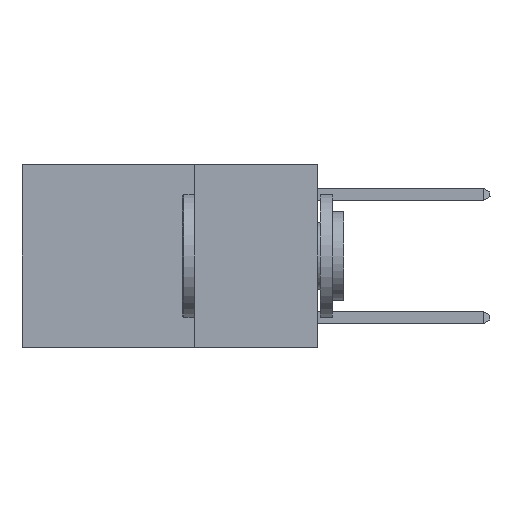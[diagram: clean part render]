
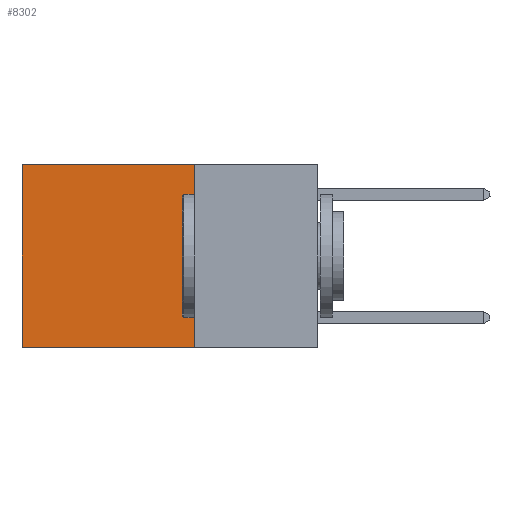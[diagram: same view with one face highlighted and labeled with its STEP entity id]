
A CAD part, left-side view. The second image highlights one B-rep face of the part: STEP entity #8302.
In plain terms, the highlighted planar face has unit normal (-1, 0, 0).
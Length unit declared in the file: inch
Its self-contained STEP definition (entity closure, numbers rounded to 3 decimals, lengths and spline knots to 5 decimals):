
#72 = LINE ( 'NONE', #10292, #3906 ) ;
#152 = VERTEX_POINT ( 'NONE', #9428 ) ;
#153 = ORIENTED_EDGE ( 'NONE', *, *, #1175, .T. ) ;
#186 = CARTESIAN_POINT ( 'NONE',  ( 0.2625, 0.6, 0. ) ) ;
#508 = CARTESIAN_POINT ( 'NONE',  ( 0.2625, 0.6, 0. ) ) ;
#593 = VERTEX_POINT ( 'NONE', #9418 ) ;
#602 = FACE_OUTER_BOUND ( 'NONE', #1276, .T. ) ;
#1175 = EDGE_CURVE ( 'NONE', #593, #5143, #72, .T. ) ;
#1276 = EDGE_LOOP ( 'NONE', ( #2510, #6364, #3151, #153 ) ) ;
#2083 = DIRECTION ( 'NONE',  ( 0., 0., -1. ) ) ;
#2302 = LINE ( 'NONE', #4546, #3843 ) ;
#2385 = DIRECTION ( 'NONE',  ( 0., 0., -1. ) ) ;
#2444 = DIRECTION ( 'NONE',  ( 1., 0., 0. ) ) ;
#2510 = ORIENTED_EDGE ( 'NONE', *, *, #2578, .T. ) ;
#2578 = EDGE_CURVE ( 'NONE', #5143, #10869, #8748, .T. ) ;
#3010 = DIRECTION ( 'NONE',  ( 0., 1., 0. ) ) ;
#3116 = LINE ( 'NONE', #4705, #4570 ) ;
#3151 = ORIENTED_EDGE ( 'NONE', *, *, #6691, .F. ) ;
#3254 = CARTESIAN_POINT ( 'NONE',  ( 0.2625, 0.25, 0. ) ) ;
#3444 = DIRECTION ( 'NONE',  ( 0., 1., 0. ) ) ;
#3843 = VECTOR ( 'NONE', #3010, 39.37008 ) ;
#3906 = VECTOR ( 'NONE', #3444, 39.37008 ) ;
#4546 = CARTESIAN_POINT ( 'NONE',  ( 0.2625, 0.25, -0.37 ) ) ;
#4570 = VECTOR ( 'NONE', #2083, 39.37008 ) ;
#4705 = CARTESIAN_POINT ( 'NONE',  ( 0.2625, 0.25, 0. ) ) ;
#5143 = VERTEX_POINT ( 'NONE', #186 ) ;
#5356 = EDGE_CURVE ( 'NONE', #152, #10869, #2302, .T. ) ;
#6364 = ORIENTED_EDGE ( 'NONE', *, *, #5356, .F. ) ;
#6392 = CARTESIAN_POINT ( 'NONE',  ( 0.2625, 0.6, -0.37 ) ) ;
#6691 = EDGE_CURVE ( 'NONE', #593, #152, #3116, .T. ) ;
#8164 = PLANE ( 'NONE',  #10051 ) ;
#8302 = ADVANCED_FACE ( 'NONE', ( #602 ), #8164, .F. ) ;
#8748 = LINE ( 'NONE', #508, #9590 ) ;
#9418 = CARTESIAN_POINT ( 'NONE',  ( 0.2625, 0.25, 0. ) ) ;
#9428 = CARTESIAN_POINT ( 'NONE',  ( 0.2625, 0.25, -0.37 ) ) ;
#9590 = VECTOR ( 'NONE', #9733, 39.37008 ) ;
#9733 = DIRECTION ( 'NONE',  ( 0., 0., -1. ) ) ;
#10051 = AXIS2_PLACEMENT_3D ( 'NONE', #3254, #2444, #2385 ) ;
#10292 = CARTESIAN_POINT ( 'NONE',  ( 0.2625, 0.25, 0. ) ) ;
#10869 = VERTEX_POINT ( 'NONE', #6392 ) ;
